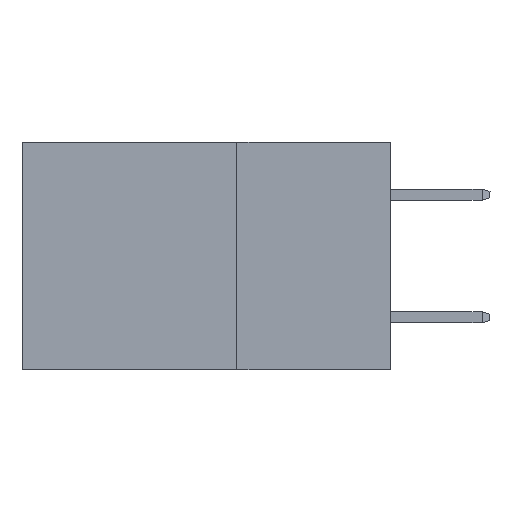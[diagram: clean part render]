
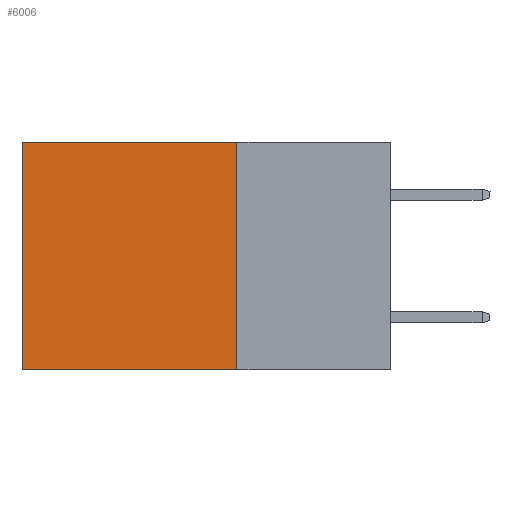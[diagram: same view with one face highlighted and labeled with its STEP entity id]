
A CAD part, left-side view. The second image highlights one B-rep face of the part: STEP entity #6006.
In plain terms, the highlighted planar face has unit normal (-1, 0, 0).
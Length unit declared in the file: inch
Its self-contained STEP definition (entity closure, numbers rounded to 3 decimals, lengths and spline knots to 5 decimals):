
#124 = CARTESIAN_POINT ( 'NONE',  ( 0.2875, 0.25, 0. ) ) ;
#171 = VERTEX_POINT ( 'NONE', #8048 ) ;
#249 = PLANE ( 'NONE',  #4065 ) ;
#431 = CARTESIAN_POINT ( 'NONE',  ( 0.2875, 0.6, 0. ) ) ;
#637 = VECTOR ( 'NONE', #1492, 39.37008 ) ;
#756 = DIRECTION ( 'NONE',  ( 0., 0., -1. ) ) ;
#1176 = VERTEX_POINT ( 'NONE', #2949 ) ;
#1492 = DIRECTION ( 'NONE',  ( 0., 1., 0. ) ) ;
#1526 = DIRECTION ( 'NONE',  ( 1., 0., 0. ) ) ;
#1565 = DIRECTION ( 'NONE',  ( 0., 0., -1. ) ) ;
#1779 = ORIENTED_EDGE ( 'NONE', *, *, #5920, .T. ) ;
#1810 = ORIENTED_EDGE ( 'NONE', *, *, #5587, .F. ) ;
#1820 = ORIENTED_EDGE ( 'NONE', *, *, #6678, .F. ) ;
#1829 = ORIENTED_EDGE ( 'NONE', *, *, #3300, .T. ) ;
#2518 = LINE ( 'NONE', #4450, #637 ) ;
#2572 = DIRECTION ( 'NONE',  ( 0., 0., -1. ) ) ;
#2949 = CARTESIAN_POINT ( 'NONE',  ( 0.2875, 0.25, -0.37 ) ) ;
#3300 = EDGE_CURVE ( 'NONE', #5583, #171, #2518, .T. ) ;
#4065 = AXIS2_PLACEMENT_3D ( 'NONE', #124, #1526, #1565 ) ;
#4120 = DIRECTION ( 'NONE',  ( 0., 1., 0. ) ) ;
#4219 = EDGE_LOOP ( 'NONE', ( #1779, #1810, #1820, #1829 ) ) ;
#4450 = CARTESIAN_POINT ( 'NONE',  ( 0.2875, 0.25, 0. ) ) ;
#5038 = CARTESIAN_POINT ( 'NONE',  ( 0.2875, 0.6, -0.37 ) ) ;
#5258 = LINE ( 'NONE', #431, #6751 ) ;
#5536 = CARTESIAN_POINT ( 'NONE',  ( 0.2875, 0.25, -0.37 ) ) ;
#5542 = VERTEX_POINT ( 'NONE', #5038 ) ;
#5563 = CARTESIAN_POINT ( 'NONE',  ( 0.2875, 0.25, 0. ) ) ;
#5583 = VERTEX_POINT ( 'NONE', #5563 ) ;
#5587 = EDGE_CURVE ( 'NONE', #1176, #5542, #8716, .T. ) ;
#5612 = FACE_OUTER_BOUND ( 'NONE', #4219, .T. ) ;
#5920 = EDGE_CURVE ( 'NONE', #171, #5542, #5258, .T. ) ;
#6006 = ADVANCED_FACE ( 'NONE', ( #5612 ), #249, .F. ) ;
#6678 = EDGE_CURVE ( 'NONE', #5583, #1176, #6839, .T. ) ;
#6751 = VECTOR ( 'NONE', #2572, 39.37008 ) ;
#6839 = LINE ( 'NONE', #8420, #8405 ) ;
#6983 = VECTOR ( 'NONE', #4120, 39.37008 ) ;
#8048 = CARTESIAN_POINT ( 'NONE',  ( 0.2875, 0.6, 0. ) ) ;
#8405 = VECTOR ( 'NONE', #756, 39.37008 ) ;
#8420 = CARTESIAN_POINT ( 'NONE',  ( 0.2875, 0.25, 0. ) ) ;
#8716 = LINE ( 'NONE', #5536, #6983 ) ;
